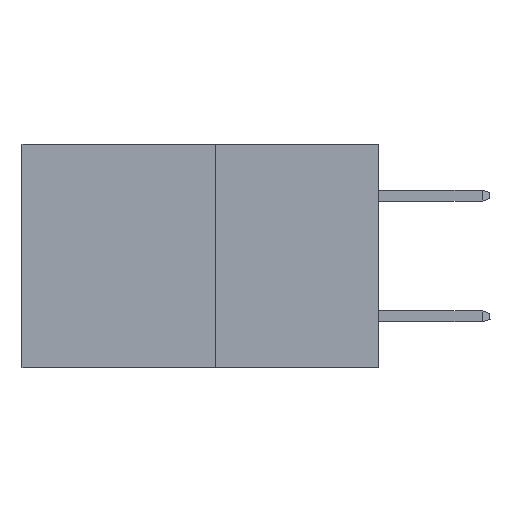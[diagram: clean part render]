
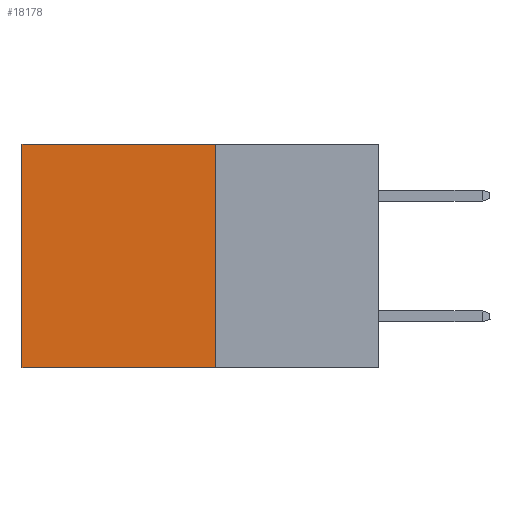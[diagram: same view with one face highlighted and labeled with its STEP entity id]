
A CAD part, left-side view. The second image highlights one B-rep face of the part: STEP entity #18178.
In plain terms, the highlighted planar face has unit normal (-1, 0, 0).
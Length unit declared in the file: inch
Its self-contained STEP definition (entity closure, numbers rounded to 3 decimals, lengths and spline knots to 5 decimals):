
#163 = CARTESIAN_POINT ( 'NONE',  ( 0.277, 0.27, 0. ) ) ;
#1347 = DIRECTION ( 'NONE',  ( 0., 0., -1. ) ) ;
#2461 = VECTOR ( 'NONE', #13033, 39.37008 ) ;
#3579 = VECTOR ( 'NONE', #9880, 39.37008 ) ;
#4104 = DIRECTION ( 'NONE',  ( 0., 0., -1. ) ) ;
#4337 = LINE ( 'NONE', #163, #3579 ) ;
#4394 = CARTESIAN_POINT ( 'NONE',  ( 0.277, 0.27, -0.37 ) ) ;
#5247 = EDGE_LOOP ( 'NONE', ( #11406, #14359, #10259, #9820 ) ) ;
#6402 = VERTEX_POINT ( 'NONE', #26542 ) ;
#6759 = VERTEX_POINT ( 'NONE', #9913 ) ;
#7598 = LINE ( 'NONE', #16300, #13294 ) ;
#8263 = PLANE ( 'NONE',  #8762 ) ;
#8527 = FACE_OUTER_BOUND ( 'NONE', #5247, .T. ) ;
#8762 = AXIS2_PLACEMENT_3D ( 'NONE', #15633, #16007, #1347 ) ;
#9820 = ORIENTED_EDGE ( 'NONE', *, *, #26817, .T. ) ;
#9880 = DIRECTION ( 'NONE',  ( 0., 1., 0. ) ) ;
#9913 = CARTESIAN_POINT ( 'NONE',  ( 0.277, 0.59, 0. ) ) ;
#10259 = ORIENTED_EDGE ( 'NONE', *, *, #30094, .F. ) ;
#11406 = ORIENTED_EDGE ( 'NONE', *, *, #24266, .T. ) ;
#13033 = DIRECTION ( 'NONE',  ( 0., 1., 0. ) ) ;
#13294 = VECTOR ( 'NONE', #4104, 39.37008 ) ;
#14359 = ORIENTED_EDGE ( 'NONE', *, *, #23288, .F. ) ;
#15633 = CARTESIAN_POINT ( 'NONE',  ( 0.277, 0.27, -0.37 ) ) ;
#16007 = DIRECTION ( 'NONE',  ( 1., 0., 0. ) ) ;
#16300 = CARTESIAN_POINT ( 'NONE',  ( 0.277, 0.27, -0.37 ) ) ;
#18178 = ADVANCED_FACE ( 'NONE', ( #8527 ), #8263, .F. ) ;
#19412 = CARTESIAN_POINT ( 'NONE',  ( 0.277, 0.59, -0.37 ) ) ;
#20248 = CARTESIAN_POINT ( 'NONE',  ( 0.277, 0.59, -0.37 ) ) ;
#21829 = DIRECTION ( 'NONE',  ( 0., 0., -1. ) ) ;
#21953 = LINE ( 'NONE', #22848, #2461 ) ;
#22664 = LINE ( 'NONE', #19412, #26881 ) ;
#22848 = CARTESIAN_POINT ( 'NONE',  ( 0.277, 0.27, -0.37 ) ) ;
#23288 = EDGE_CURVE ( 'NONE', #27299, #23938, #21953, .T. ) ;
#23938 = VERTEX_POINT ( 'NONE', #20248 ) ;
#24266 = EDGE_CURVE ( 'NONE', #6759, #23938, #22664, .T. ) ;
#26542 = CARTESIAN_POINT ( 'NONE',  ( 0.277, 0.27, 0. ) ) ;
#26817 = EDGE_CURVE ( 'NONE', #6402, #6759, #4337, .T. ) ;
#26881 = VECTOR ( 'NONE', #21829, 39.37008 ) ;
#27299 = VERTEX_POINT ( 'NONE', #4394 ) ;
#30094 = EDGE_CURVE ( 'NONE', #6402, #27299, #7598, .T. ) ;
